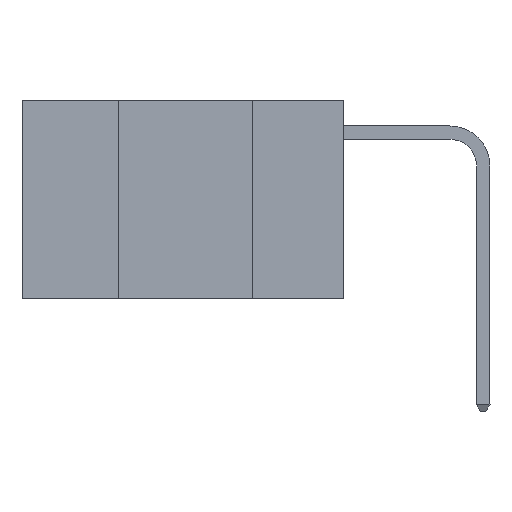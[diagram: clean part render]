
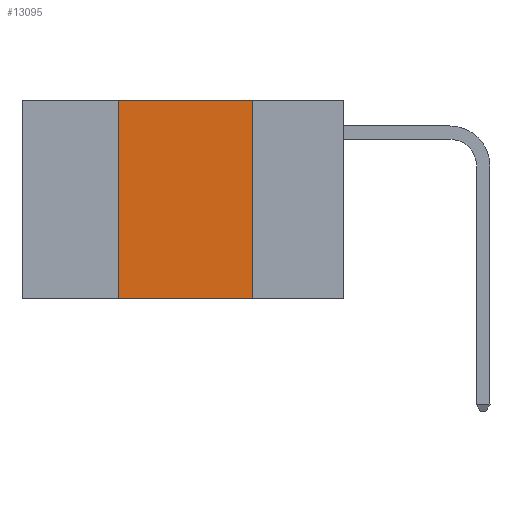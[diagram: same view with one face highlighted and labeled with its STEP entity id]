
A CAD part, left-side view. The second image highlights one B-rep face of the part: STEP entity #13095.
In plain terms, the highlighted planar face has unit normal (-1, 0, 0).
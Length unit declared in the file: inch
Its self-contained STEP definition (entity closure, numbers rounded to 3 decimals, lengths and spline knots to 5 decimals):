
#61 = CARTESIAN_POINT ( 'NONE',  ( 0., 0.42, 0. ) ) ;
#1012 = CARTESIAN_POINT ( 'NONE',  ( 0., 0.17, 0. ) ) ;
#1633 = AXIS2_PLACEMENT_3D ( 'NONE', #3248, #13552, #5887 ) ;
#2301 = CARTESIAN_POINT ( 'NONE',  ( 0., 0.17, 0. ) ) ;
#3171 = ORIENTED_EDGE ( 'NONE', *, *, #16586, .F. ) ;
#3248 = CARTESIAN_POINT ( 'NONE',  ( 0., 0.6, 0. ) ) ;
#3304 = LINE ( 'NONE', #2301, #16606 ) ;
#3846 = VECTOR ( 'NONE', #12755, 39.37008 ) ;
#4701 = EDGE_CURVE ( 'NONE', #12453, #5619, #11862, .T. ) ;
#4718 = LINE ( 'NONE', #8673, #5141 ) ;
#5027 = VERTEX_POINT ( 'NONE', #1012 ) ;
#5141 = VECTOR ( 'NONE', #11225, 39.37008 ) ;
#5619 = VERTEX_POINT ( 'NONE', #61 ) ;
#5887 = DIRECTION ( 'NONE',  ( 0., 0., -1. ) ) ;
#6303 = CARTESIAN_POINT ( 'NONE',  ( 0., 0.6, 0. ) ) ;
#6790 = CARTESIAN_POINT ( 'NONE',  ( 0., 0.17, -0.37 ) ) ;
#7555 = VERTEX_POINT ( 'NONE', #6790 ) ;
#7891 = EDGE_CURVE ( 'NONE', #5027, #7555, #3304, .T. ) ;
#8673 = CARTESIAN_POINT ( 'NONE',  ( 0., 0.6, -0.37 ) ) ;
#9526 = EDGE_CURVE ( 'NONE', #12453, #7555, #4718, .T. ) ;
#10086 = DIRECTION ( 'NONE',  ( 0., 0., -1. ) ) ;
#10684 = LINE ( 'NONE', #6303, #3846 ) ;
#10997 = PLANE ( 'NONE',  #1633 ) ;
#11000 = EDGE_LOOP ( 'NONE', ( #12817, #3171, #15441, #16073 ) ) ;
#11225 = DIRECTION ( 'NONE',  ( 0., -1., 0. ) ) ;
#11862 = LINE ( 'NONE', #12195, #14846 ) ;
#12195 = CARTESIAN_POINT ( 'NONE',  ( 0., 0.42, 0. ) ) ;
#12248 = CARTESIAN_POINT ( 'NONE',  ( 0., 0.42, -0.37 ) ) ;
#12453 = VERTEX_POINT ( 'NONE', #12248 ) ;
#12755 = DIRECTION ( 'NONE',  ( 0., -1., 0. ) ) ;
#12817 = ORIENTED_EDGE ( 'NONE', *, *, #7891, .F. ) ;
#13095 = ADVANCED_FACE ( 'NONE', ( #16192 ), #10997, .F. ) ;
#13467 = DIRECTION ( 'NONE',  ( 0., 0., 1. ) ) ;
#13552 = DIRECTION ( 'NONE',  ( 1., 0., 0. ) ) ;
#14846 = VECTOR ( 'NONE', #13467, 39.37008 ) ;
#15441 = ORIENTED_EDGE ( 'NONE', *, *, #4701, .F. ) ;
#16073 = ORIENTED_EDGE ( 'NONE', *, *, #9526, .T. ) ;
#16192 = FACE_OUTER_BOUND ( 'NONE', #11000, .T. ) ;
#16586 = EDGE_CURVE ( 'NONE', #5619, #5027, #10684, .T. ) ;
#16606 = VECTOR ( 'NONE', #10086, 39.37008 ) ;
